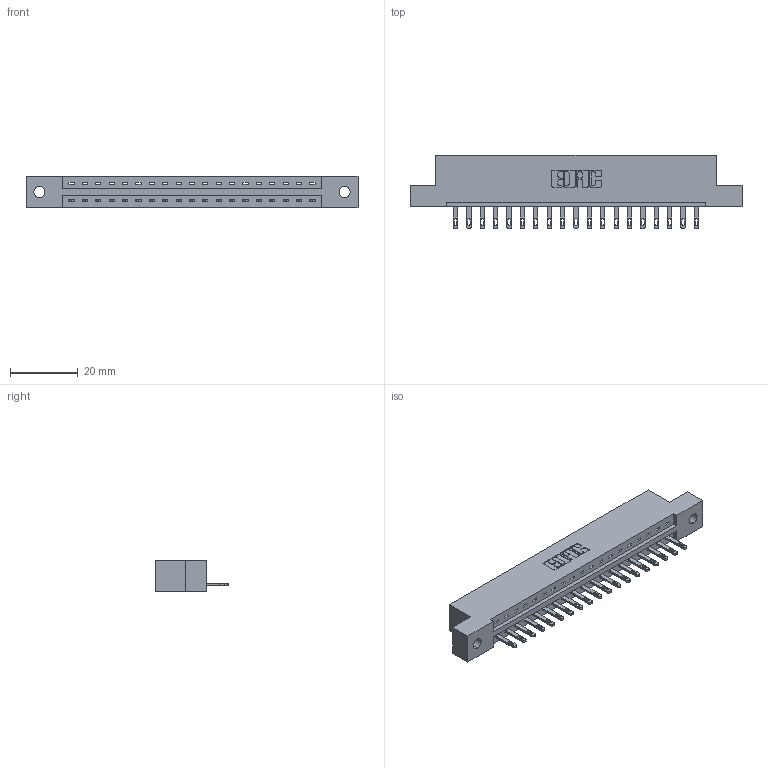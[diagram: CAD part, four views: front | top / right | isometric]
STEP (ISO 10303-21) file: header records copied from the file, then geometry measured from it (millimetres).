
FILE_DESCRIPTION (( 'STEP AP203' ), '1' );
FILE_NAME ('887-019-500-102.STEP', '2020-09-20T17:52:41', ( '' ), ( '' ), 'SwSTEP 2.0', 'SolidWorks 2020', '' );
FILE_SCHEMA (( 'CONFIG_CONTROL_DESIGN' ));
Length unit declared in the file: inch
Products named in the file (3): 837 Part_Flush Mounting Lugs - 0.128 Dia; 887-019-500-102; 345-292-001_345-293-100
Assembly tree (20 placements, depth 2):
  887-019-500-102
    837 Part_Flush Mounting Lugs - 0.128 Dia
    345-292-001_345-293-100  x19
Bounding box: 98.3 x 21.85 x 9.4 mm (x, y, z)
Volume: 9903.7 mm3; surface area: 9880.8 mm2
Topology: 20 solids, 20 shells, 1216 faces, 3731 edges, 2486 vertices
Faces by surface type: plane 830, cylinder 386
Entity records: 17031 total; most frequent: CARTESIAN_POINT 2971, ORIENTED_EDGE 2926, DIRECTION 2549, EDGE_CURVE 1463, LINE 1331, VECTOR 1331, VERTEX_POINT 974, AXIS2_PLACEMENT_3D 609
